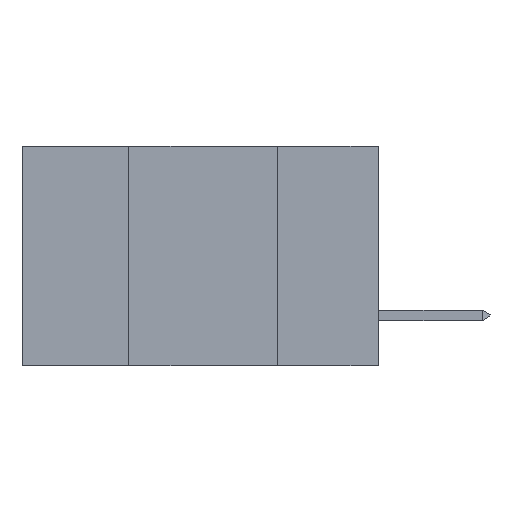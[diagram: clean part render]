
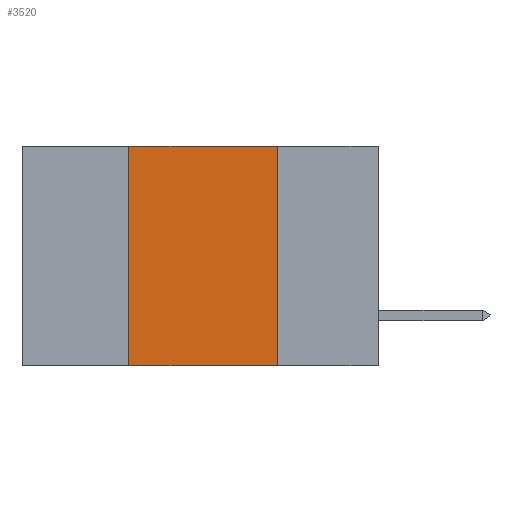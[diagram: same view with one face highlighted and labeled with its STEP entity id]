
A CAD part, left-side view. The second image highlights one B-rep face of the part: STEP entity #3520.
In plain terms, the highlighted planar face has unit normal (-1, 0, 0).
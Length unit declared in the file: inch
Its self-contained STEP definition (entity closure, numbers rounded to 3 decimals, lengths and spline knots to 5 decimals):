
#1040 = CARTESIAN_POINT ( 'NONE',  ( 0., 0.6, -0.37 ) ) ;
#2006 = CARTESIAN_POINT ( 'NONE',  ( 0., 0.42, 0. ) ) ;
#2752 = CARTESIAN_POINT ( 'NONE',  ( 0., 0.42, -0.37 ) ) ;
#3170 = EDGE_CURVE ( 'NONE', #20555, #17819, #7803, .T. ) ;
#3520 = ADVANCED_FACE ( 'NONE', ( #15792 ), #17443, .F. ) ;
#3764 = DIRECTION ( 'NONE',  ( 0., 0., -1. ) ) ;
#4149 = VECTOR ( 'NONE', #19939, 39.37008 ) ;
#4439 = CARTESIAN_POINT ( 'NONE',  ( 0., 0.17, 0. ) ) ;
#4756 = DIRECTION ( 'NONE',  ( 0., -1., 0. ) ) ;
#5298 = CARTESIAN_POINT ( 'NONE',  ( 0., 0.6, 0. ) ) ;
#5399 = CARTESIAN_POINT ( 'NONE',  ( 0., 0.6, 0. ) ) ;
#5620 = DIRECTION ( 'NONE',  ( 1., 0., 0. ) ) ;
#5859 = EDGE_LOOP ( 'NONE', ( #9165, #6254, #6096, #14295 ) ) ;
#6096 = ORIENTED_EDGE ( 'NONE', *, *, #9894, .F. ) ;
#6254 = ORIENTED_EDGE ( 'NONE', *, *, #17915, .F. ) ;
#7803 = LINE ( 'NONE', #1040, #17323 ) ;
#8455 = LINE ( 'NONE', #18513, #4149 ) ;
#8629 = CARTESIAN_POINT ( 'NONE',  ( 0., 0.42, -0.37 ) ) ;
#9165 = ORIENTED_EDGE ( 'NONE', *, *, #14257, .F. ) ;
#9894 = EDGE_CURVE ( 'NONE', #20555, #19586, #14691, .T. ) ;
#11162 = DIRECTION ( 'NONE',  ( 0., 0., 1. ) ) ;
#11954 = DIRECTION ( 'NONE',  ( 0., -1., 0. ) ) ;
#12003 = AXIS2_PLACEMENT_3D ( 'NONE', #5399, #5620, #3764 ) ;
#14257 = EDGE_CURVE ( 'NONE', #15344, #17819, #8455, .T. ) ;
#14295 = ORIENTED_EDGE ( 'NONE', *, *, #3170, .T. ) ;
#14691 = LINE ( 'NONE', #2752, #20429 ) ;
#15344 = VERTEX_POINT ( 'NONE', #4439 ) ;
#15792 = FACE_OUTER_BOUND ( 'NONE', #5859, .T. ) ;
#17128 = CARTESIAN_POINT ( 'NONE',  ( 0., 0.17, -0.37 ) ) ;
#17323 = VECTOR ( 'NONE', #4756, 39.37008 ) ;
#17443 = PLANE ( 'NONE',  #12003 ) ;
#17819 = VERTEX_POINT ( 'NONE', #17128 ) ;
#17915 = EDGE_CURVE ( 'NONE', #19586, #15344, #20292, .T. ) ;
#18177 = VECTOR ( 'NONE', #11954, 39.37008 ) ;
#18513 = CARTESIAN_POINT ( 'NONE',  ( 0., 0.17, -0.37 ) ) ;
#19586 = VERTEX_POINT ( 'NONE', #2006 ) ;
#19939 = DIRECTION ( 'NONE',  ( 0., 0., -1. ) ) ;
#20292 = LINE ( 'NONE', #5298, #18177 ) ;
#20429 = VECTOR ( 'NONE', #11162, 39.37008 ) ;
#20555 = VERTEX_POINT ( 'NONE', #8629 ) ;
